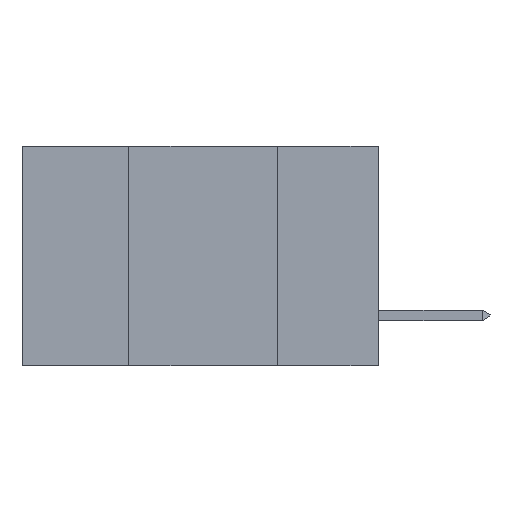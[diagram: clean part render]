
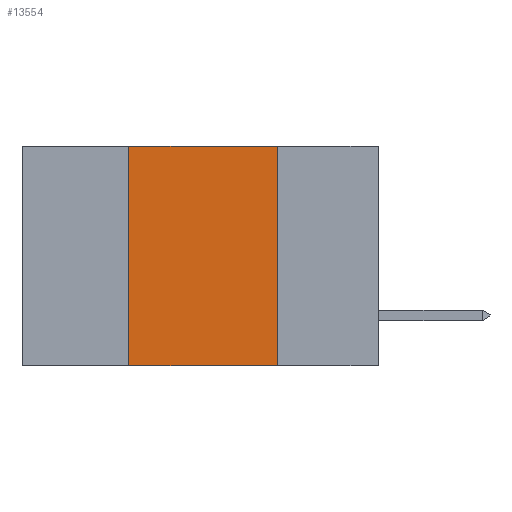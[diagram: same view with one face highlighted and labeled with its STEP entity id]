
A CAD part, left-side view. The second image highlights one B-rep face of the part: STEP entity #13554.
In plain terms, the highlighted planar face has unit normal (-1, 0, 0).
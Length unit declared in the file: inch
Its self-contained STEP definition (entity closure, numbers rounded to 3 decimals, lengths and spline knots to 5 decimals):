
#245 = AXIS2_PLACEMENT_3D ( 'NONE', #7288, #1461, #17493 ) ;
#1461 = DIRECTION ( 'NONE',  ( 1., 0., 0. ) ) ;
#3175 = ORIENTED_EDGE ( 'NONE', *, *, #16632, .F. ) ;
#3395 = CARTESIAN_POINT ( 'NONE',  ( 0., 0.17, -0.37 ) ) ;
#4473 = DIRECTION ( 'NONE',  ( 0., 0., 1. ) ) ;
#4981 = CARTESIAN_POINT ( 'NONE',  ( 0., 0.42, 0. ) ) ;
#5093 = VERTEX_POINT ( 'NONE', #11918 ) ;
#5111 = VERTEX_POINT ( 'NONE', #7555 ) ;
#5701 = DIRECTION ( 'NONE',  ( 0., -1., 0. ) ) ;
#5810 = VERTEX_POINT ( 'NONE', #4981 ) ;
#6978 = VECTOR ( 'NONE', #5701, 39.37008 ) ;
#7288 = CARTESIAN_POINT ( 'NONE',  ( 0., 0.6, 0. ) ) ;
#7555 = CARTESIAN_POINT ( 'NONE',  ( 0., 0.42, -0.37 ) ) ;
#9262 = EDGE_LOOP ( 'NONE', ( #13655, #22533, #3175, #24468 ) ) ;
#9688 = CARTESIAN_POINT ( 'NONE',  ( 0., 0.6, -0.37 ) ) ;
#9908 = EDGE_CURVE ( 'NONE', #5093, #11939, #12356, .T. ) ;
#11406 = PLANE ( 'NONE',  #245 ) ;
#11655 = LINE ( 'NONE', #9688, #6978 ) ;
#11918 = CARTESIAN_POINT ( 'NONE',  ( 0., 0.17, 0. ) ) ;
#11939 = VERTEX_POINT ( 'NONE', #3395 ) ;
#12088 = LINE ( 'NONE', #20190, #24455 ) ;
#12301 = VECTOR ( 'NONE', #24404, 39.37008 ) ;
#12356 = LINE ( 'NONE', #22438, #12301 ) ;
#12541 = LINE ( 'NONE', #20642, #23576 ) ;
#13554 = ADVANCED_FACE ( 'NONE', ( #25165 ), #11406, .F. ) ;
#13655 = ORIENTED_EDGE ( 'NONE', *, *, #9908, .F. ) ;
#16632 = EDGE_CURVE ( 'NONE', #5111, #5810, #12541, .T. ) ;
#17493 = DIRECTION ( 'NONE',  ( 0., 0., -1. ) ) ;
#17821 = EDGE_CURVE ( 'NONE', #5810, #5093, #12088, .T. ) ;
#20190 = CARTESIAN_POINT ( 'NONE',  ( 0., 0.6, 0. ) ) ;
#20642 = CARTESIAN_POINT ( 'NONE',  ( 0., 0.42, -0.37 ) ) ;
#22438 = CARTESIAN_POINT ( 'NONE',  ( 0., 0.17, -0.37 ) ) ;
#22533 = ORIENTED_EDGE ( 'NONE', *, *, #17821, .F. ) ;
#23576 = VECTOR ( 'NONE', #4473, 39.37008 ) ;
#24135 = EDGE_CURVE ( 'NONE', #5111, #11939, #11655, .T. ) ;
#24387 = DIRECTION ( 'NONE',  ( 0., -1., 0. ) ) ;
#24404 = DIRECTION ( 'NONE',  ( 0., 0., -1. ) ) ;
#24455 = VECTOR ( 'NONE', #24387, 39.37008 ) ;
#24468 = ORIENTED_EDGE ( 'NONE', *, *, #24135, .T. ) ;
#25165 = FACE_OUTER_BOUND ( 'NONE', #9262, .T. ) ;
